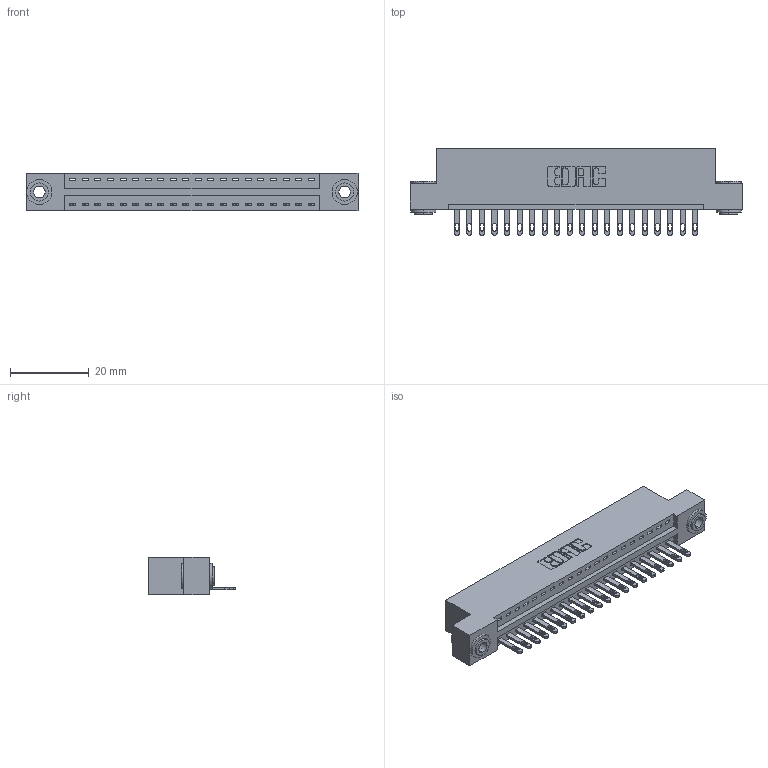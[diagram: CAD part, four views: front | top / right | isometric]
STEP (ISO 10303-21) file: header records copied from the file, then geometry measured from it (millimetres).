
FILE_DESCRIPTION (( 'STEP AP203' ), '1' );
FILE_NAME ('896-020-500-103.STEP', '2021-07-27T16:27:23', ( '' ), ( '' ), 'SwSTEP 2.0', 'SolidWorks 2020', '' );
FILE_SCHEMA (( 'CONFIG_CONTROL_DESIGN' ));
Length unit declared in the file: inch
Products named in the file (4): 896-020-500-103; 345-292-001_345-293-100; 846 Part_Flush Mounting Lugs - 0.156 Dia-TH; 345-250-002_345-250-002-102
Assembly tree (23 placements, depth 2):
  896-020-500-103
    846 Part_Flush Mounting Lugs - 0.156 Dia-TH
    345-292-001_345-293-100  x20
    345-250-002_345-250-002-102  x2
Bounding box: 84.07 x 21.84 x 9.4 mm (x, y, z)
Volume: 7927.9 mm3; surface area: 9937.3 mm2
Topology: 23 solids, 23 shells, 1240 faces, 3765 edges, 2506 vertices
Faces by surface type: plane 766, cylinder 466, cone 8
Entity records: 15954 total; most frequent: CARTESIAN_POINT 2719, ORIENTED_EDGE 2666, DIRECTION 2459, EDGE_CURVE 1333, VECTOR 1093, LINE 1093, VERTEX_POINT 886, AXIS2_PLACEMENT_3D 683
